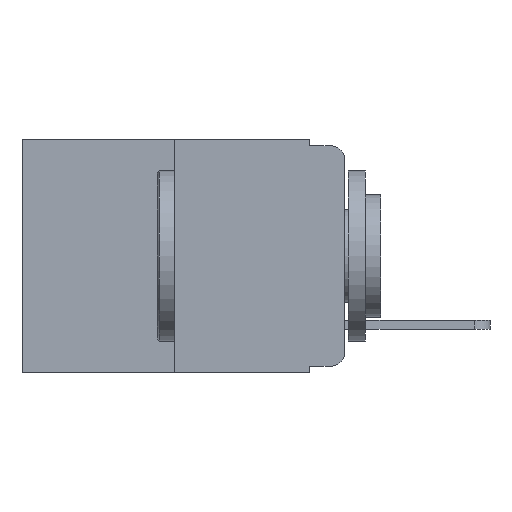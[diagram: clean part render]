
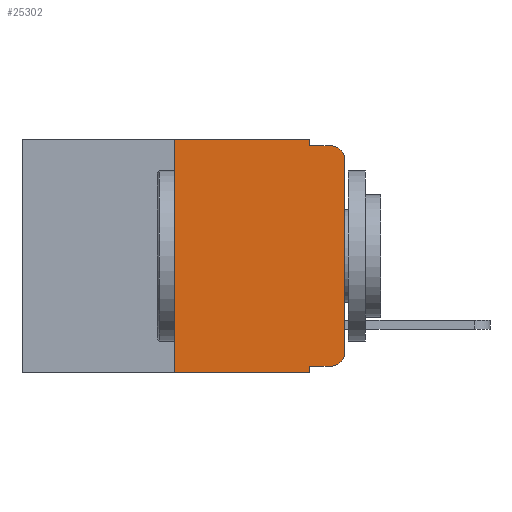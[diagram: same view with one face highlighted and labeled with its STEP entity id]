
A CAD part, left-side view. The second image highlights one B-rep face of the part: STEP entity #25302.
In plain terms, the highlighted planar face has unit normal (-1, 0, 0).
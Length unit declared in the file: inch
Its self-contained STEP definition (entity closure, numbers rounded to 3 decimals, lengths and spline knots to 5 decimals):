
#183 = ORIENTED_EDGE ( 'NONE', *, *, #23696, .T. ) ;
#265 = CARTESIAN_POINT ( 'NONE',  ( 0., 0.25, 0. ) ) ;
#296 = DIRECTION ( 'NONE',  ( 0., 0., -1. ) ) ;
#424 = LINE ( 'NONE', #17776, #21157 ) ;
#524 = DIRECTION ( 'NONE',  ( 0., -1., 0. ) ) ;
#1240 = EDGE_CURVE ( 'NONE', #13574, #18169, #18407, .T. ) ;
#1878 = CARTESIAN_POINT ( 'NONE',  ( 0., 0.051, 0. ) ) ;
#2582 = CARTESIAN_POINT ( 'NONE',  ( 0., 0.051, -0.01 ) ) ;
#3063 = VECTOR ( 'NONE', #20702, 39.37008 ) ;
#3556 = EDGE_CURVE ( 'NONE', #24390, #19149, #15318, .T. ) ;
#3752 = CARTESIAN_POINT ( 'NONE',  ( 0., 0.25, -0.343 ) ) ;
#3946 = LINE ( 'NONE', #25806, #11648 ) ;
#4553 = CARTESIAN_POINT ( 'NONE',  ( 0., 0.051, -0.01 ) ) ;
#4555 = CARTESIAN_POINT ( 'NONE',  ( 0., 0.02, -0.313 ) ) ;
#4888 = VECTOR ( 'NONE', #10681, 39.37008 ) ;
#5714 = VERTEX_POINT ( 'NONE', #16992 ) ;
#5802 = ORIENTED_EDGE ( 'NONE', *, *, #13791, .F. ) ;
#6023 = AXIS2_PLACEMENT_3D ( 'NONE', #11439, #13353, #21850 ) ;
#6286 = CARTESIAN_POINT ( 'NONE',  ( 0., 0., -0.03 ) ) ;
#6414 = FACE_OUTER_BOUND ( 'NONE', #25894, .T. ) ;
#6611 = EDGE_CURVE ( 'NONE', #26439, #24390, #25824, .T. ) ;
#7332 = DIRECTION ( 'NONE',  ( 0., 0., -1. ) ) ;
#9206 = DIRECTION ( 'NONE',  ( 0., 0., 1. ) ) ;
#10216 = CARTESIAN_POINT ( 'NONE',  ( 0., 0.02, -0.333 ) ) ;
#10601 = DIRECTION ( 'NONE',  ( 0., -1., 0. ) ) ;
#10681 = DIRECTION ( 'NONE',  ( 0., -1., 0. ) ) ;
#10780 = DIRECTION ( 'NONE',  ( -1., 0., 0. ) ) ;
#11439 = CARTESIAN_POINT ( 'NONE',  ( 0., 0.473, 0. ) ) ;
#11648 = VECTOR ( 'NONE', #9206, 39.37008 ) ;
#12159 = DIRECTION ( 'NONE',  ( 0., -1., 0. ) ) ;
#12249 = ORIENTED_EDGE ( 'NONE', *, *, #15031, .T. ) ;
#12517 = LINE ( 'NONE', #4553, #24504 ) ;
#12587 = DIRECTION ( 'NONE',  ( -1., 0., 0. ) ) ;
#12621 = ORIENTED_EDGE ( 'NONE', *, *, #1240, .F. ) ;
#12748 = AXIS2_PLACEMENT_3D ( 'NONE', #4555, #10780, #296 ) ;
#12817 = EDGE_CURVE ( 'NONE', #21872, #14845, #424, .T. ) ;
#13353 = DIRECTION ( 'NONE',  ( 1., 0., 0. ) ) ;
#13574 = VERTEX_POINT ( 'NONE', #3752 ) ;
#13724 = VERTEX_POINT ( 'NONE', #6286 ) ;
#13791 = EDGE_CURVE ( 'NONE', #18169, #21872, #13953, .T. ) ;
#13953 = LINE ( 'NONE', #22906, #4888 ) ;
#14583 = ORIENTED_EDGE ( 'NONE', *, *, #3556, .T. ) ;
#14612 = CARTESIAN_POINT ( 'NONE',  ( 0., 0.02, -0.01 ) ) ;
#14845 = VERTEX_POINT ( 'NONE', #2582 ) ;
#14942 = ORIENTED_EDGE ( 'NONE', *, *, #12817, .F. ) ;
#14956 = CARTESIAN_POINT ( 'NONE',  ( 0., 0.25, 0. ) ) ;
#15031 = EDGE_CURVE ( 'NONE', #19149, #13724, #3946, .T. ) ;
#15318 = CIRCLE ( 'NONE', #12748, 0.02 ) ;
#15578 = PLANE ( 'NONE',  #6023 ) ;
#15844 = ORIENTED_EDGE ( 'NONE', *, *, #6611, .T. ) ;
#16208 = AXIS2_PLACEMENT_3D ( 'NONE', #24961, #12587, #16792 ) ;
#16786 = VERTEX_POINT ( 'NONE', #14612 ) ;
#16792 = DIRECTION ( 'NONE',  ( 0., 0., -1. ) ) ;
#16992 = CARTESIAN_POINT ( 'NONE',  ( 0., 0.051, -0.343 ) ) ;
#17527 = EDGE_CURVE ( 'NONE', #13724, #16786, #21389, .T. ) ;
#17776 = CARTESIAN_POINT ( 'NONE',  ( 0., 0.051, 0. ) ) ;
#17978 = EDGE_CURVE ( 'NONE', #26439, #5714, #18917, .T. ) ;
#18169 = VERTEX_POINT ( 'NONE', #14956 ) ;
#18299 = LINE ( 'NONE', #26780, #19598 ) ;
#18407 = LINE ( 'NONE', #265, #21670 ) ;
#18917 = LINE ( 'NONE', #1878, #3063 ) ;
#19149 = VERTEX_POINT ( 'NONE', #26748 ) ;
#19542 = CARTESIAN_POINT ( 'NONE',  ( 0., 0.051, -0.333 ) ) ;
#19598 = VECTOR ( 'NONE', #12159, 39.37008 ) ;
#20603 = ORIENTED_EDGE ( 'NONE', *, *, #25679, .F. ) ;
#20629 = DIRECTION ( 'NONE',  ( 0., 0., 1. ) ) ;
#20702 = DIRECTION ( 'NONE',  ( 0., 0., -1. ) ) ;
#20813 = CARTESIAN_POINT ( 'NONE',  ( 0., 0.051, 0. ) ) ;
#21157 = VECTOR ( 'NONE', #7332, 39.37008 ) ;
#21389 = CIRCLE ( 'NONE', #16208, 0.02 ) ;
#21573 = ORIENTED_EDGE ( 'NONE', *, *, #17978, .F. ) ;
#21670 = VECTOR ( 'NONE', #20629, 39.37008 ) ;
#21850 = DIRECTION ( 'NONE',  ( 0., 0., -1. ) ) ;
#21872 = VERTEX_POINT ( 'NONE', #20813 ) ;
#22906 = CARTESIAN_POINT ( 'NONE',  ( 0., 0.473, 0. ) ) ;
#23226 = CARTESIAN_POINT ( 'NONE',  ( 0., 0.051, -0.333 ) ) ;
#23257 = VECTOR ( 'NONE', #524, 39.37008 ) ;
#23388 = ORIENTED_EDGE ( 'NONE', *, *, #17527, .T. ) ;
#23696 = EDGE_CURVE ( 'NONE', #13574, #5714, #18299, .T. ) ;
#24390 = VERTEX_POINT ( 'NONE', #10216 ) ;
#24504 = VECTOR ( 'NONE', #10601, 39.37008 ) ;
#24961 = CARTESIAN_POINT ( 'NONE',  ( 0., 0.02, -0.03 ) ) ;
#25302 = ADVANCED_FACE ( 'NONE', ( #6414 ), #15578, .F. ) ;
#25679 = EDGE_CURVE ( 'NONE', #14845, #16786, #12517, .T. ) ;
#25806 = CARTESIAN_POINT ( 'NONE',  ( 0., 0., 0. ) ) ;
#25824 = LINE ( 'NONE', #23226, #23257 ) ;
#25894 = EDGE_LOOP ( 'NONE', ( #12249, #23388, #20603, #14942, #5802, #12621, #183, #21573, #15844, #14583 ) ) ;
#26439 = VERTEX_POINT ( 'NONE', #19542 ) ;
#26748 = CARTESIAN_POINT ( 'NONE',  ( 0., 0., -0.313 ) ) ;
#26780 = CARTESIAN_POINT ( 'NONE',  ( 0., 0.473, -0.343 ) ) ;
